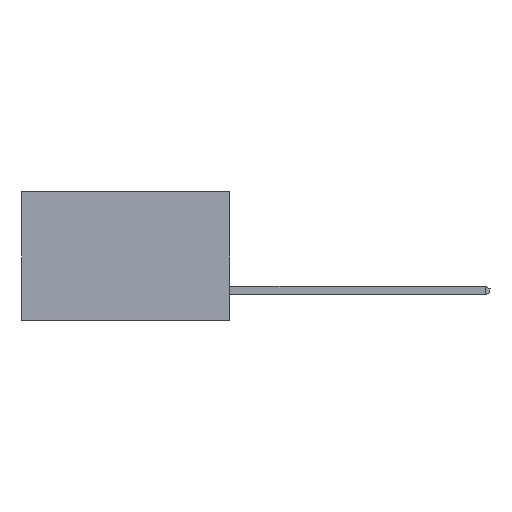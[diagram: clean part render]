
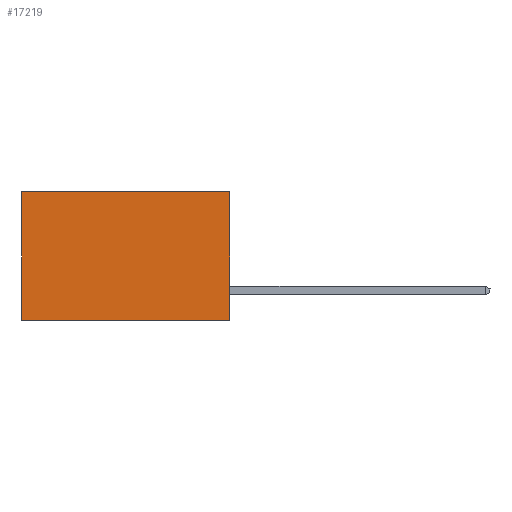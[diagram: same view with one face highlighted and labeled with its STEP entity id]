
A CAD part, left-side view. The second image highlights one B-rep face of the part: STEP entity #17219.
In plain terms, the highlighted planar face has unit normal (-1, 0, 0).
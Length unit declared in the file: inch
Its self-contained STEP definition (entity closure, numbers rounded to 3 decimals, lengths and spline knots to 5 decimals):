
#111 = ORIENTED_EDGE ( 'NONE', *, *, #23040, .T. ) ;
#218 = VERTEX_POINT ( 'NONE', #18538 ) ;
#604 = CARTESIAN_POINT ( 'NONE',  ( 0.2615, 0.6, -0.37 ) ) ;
#1598 = LINE ( 'NONE', #1959, #21421 ) ;
#1925 = CARTESIAN_POINT ( 'NONE',  ( 0.2615, 0., -0.37 ) ) ;
#1959 = CARTESIAN_POINT ( 'NONE',  ( 0.2615, 0., -0.37 ) ) ;
#2121 = EDGE_LOOP ( 'NONE', ( #111, #19779, #11290, #7034 ) ) ;
#2831 = VECTOR ( 'NONE', #11485, 39.37008 ) ;
#3560 = DIRECTION ( 'NONE',  ( 0., 0., -1. ) ) ;
#3858 = FACE_OUTER_BOUND ( 'NONE', #2121, .T. ) ;
#6156 = DIRECTION ( 'NONE',  ( 0., 0., -1. ) ) ;
#7034 = ORIENTED_EDGE ( 'NONE', *, *, #9180, .T. ) ;
#8332 = DIRECTION ( 'NONE',  ( 1., 0., 0. ) ) ;
#8435 = VERTEX_POINT ( 'NONE', #23224 ) ;
#9170 = LINE ( 'NONE', #17071, #9280 ) ;
#9180 = EDGE_CURVE ( 'NONE', #218, #8435, #13211, .T. ) ;
#9280 = VECTOR ( 'NONE', #3560, 39.37008 ) ;
#10828 = VECTOR ( 'NONE', #15133, 39.37008 ) ;
#11290 = ORIENTED_EDGE ( 'NONE', *, *, #20446, .F. ) ;
#11485 = DIRECTION ( 'NONE',  ( 0., 1., 0. ) ) ;
#12865 = EDGE_CURVE ( 'NONE', #14748, #14759, #15555, .T. ) ;
#13211 = LINE ( 'NONE', #22665, #10828 ) ;
#13321 = DIRECTION ( 'NONE',  ( 0., 0., -1. ) ) ;
#14748 = VERTEX_POINT ( 'NONE', #24898 ) ;
#14759 = VERTEX_POINT ( 'NONE', #604 ) ;
#15133 = DIRECTION ( 'NONE',  ( 0., 1., 0. ) ) ;
#15555 = LINE ( 'NONE', #1925, #2831 ) ;
#17071 = CARTESIAN_POINT ( 'NONE',  ( 0.2615, 0.6, -0.37 ) ) ;
#17219 = ADVANCED_FACE ( 'NONE', ( #3858 ), #17844, .F. ) ;
#17844 = PLANE ( 'NONE',  #19685 ) ;
#18538 = CARTESIAN_POINT ( 'NONE',  ( 0.2615, 0., 0. ) ) ;
#19685 = AXIS2_PLACEMENT_3D ( 'NONE', #23871, #8332, #6156 ) ;
#19779 = ORIENTED_EDGE ( 'NONE', *, *, #12865, .F. ) ;
#20446 = EDGE_CURVE ( 'NONE', #218, #14748, #1598, .T. ) ;
#21421 = VECTOR ( 'NONE', #13321, 39.37008 ) ;
#22665 = CARTESIAN_POINT ( 'NONE',  ( 0.2615, 0., 0. ) ) ;
#23040 = EDGE_CURVE ( 'NONE', #8435, #14759, #9170, .T. ) ;
#23224 = CARTESIAN_POINT ( 'NONE',  ( 0.2615, 0.6, 0. ) ) ;
#23871 = CARTESIAN_POINT ( 'NONE',  ( 0.2615, 0., -0.37 ) ) ;
#24898 = CARTESIAN_POINT ( 'NONE',  ( 0.2615, 0., -0.37 ) ) ;
